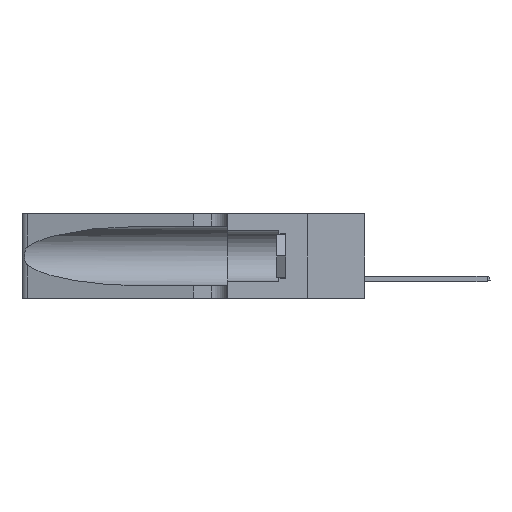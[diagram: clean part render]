
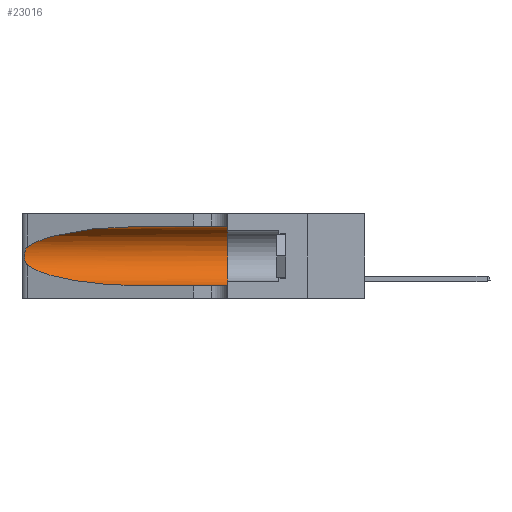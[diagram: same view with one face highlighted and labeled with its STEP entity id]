
A CAD part, left-side view. The second image highlights one B-rep face of the part: STEP entity #23016.
In plain terms, the highlighted cylindrical face has radius 3.308 mm (diameter 6.617 mm), a partial arc.
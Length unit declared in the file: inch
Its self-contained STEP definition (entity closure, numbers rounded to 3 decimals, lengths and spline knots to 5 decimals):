
#11 = EDGE_LOOP ( 'NONE', ( #14268, #11052, #5987, #9031, #28122, #39845 ) ) ;
#820 = CIRCLE ( 'NONE', #30884, 0.13025 ) ;
#2294 =( BOUNDED_CURVE ( )  B_SPLINE_CURVE ( 3, ( #7659, #23607, #17549, #39515 ),
 .UNSPECIFIED., .F., .F. ) 
 B_SPLINE_CURVE_WITH_KNOTS ( ( 4, 4 ),
 ( 1.5708, 2.84003 ),
 .UNSPECIFIED. ) 
 CURVE ( )  GEOMETRIC_REPRESENTATION_ITEM ( )  RATIONAL_B_SPLINE_CURVE ( ( 1., 0.87, 0.87, 1. ) ) 
 REPRESENTATION_ITEM ( '' )  );
#2702 = CARTESIAN_POINT ( 'NONE',  ( 0.25487, 1.22718, 0.14631 ) ) ;
#5159 = VERTEX_POINT ( 'NONE', #16169 ) ;
#5179 = CARTESIAN_POINT ( 'NONE',  ( 0.2373, 1.15595, 0.08982 ) ) ;
#5259 = CARTESIAN_POINT ( 'NONE',  ( 0.1305, 0.35, 0.185 ) ) ;
#5987 = ORIENTED_EDGE ( 'NONE', *, *, #15697, .T. ) ;
#7659 = CARTESIAN_POINT ( 'NONE',  ( 0.1305, 0.72297, 0.31525 ) ) ;
#9031 = ORIENTED_EDGE ( 'NONE', *, *, #18591, .T. ) ;
#10205 = CARTESIAN_POINT ( 'NONE',  ( 0.1305, 0.35, 0.31525 ) ) ;
#11052 = ORIENTED_EDGE ( 'NONE', *, *, #32203, .T. ) ;
#11164 = DIRECTION ( 'NONE',  ( 0., -1., 0. ) ) ;
#11564 = DIRECTION ( 'NONE',  ( 0., 0., 1. ) ) ;
#11741 = CARTESIAN_POINT ( 'NONE',  ( 0.25555, 1.22994, 0.2215 ) ) ;
#11879 = CARTESIAN_POINT ( 'NONE',  ( 0.25487, 1.22718, 0.22369 ) ) ;
#12000 = CARTESIAN_POINT ( 'NONE',  ( 0.26017, 1.23833, 0.17102 ) ) ;
#12102 = CARTESIAN_POINT ( 'NONE',  ( 0.1305, 1.61858, 0.31525 ) ) ;
#12310 = LINE ( 'NONE', #12102, #27990 ) ;
#13757 = CARTESIAN_POINT ( 'NONE',  ( 0.1305, 1.61858, 0.185 ) ) ;
#14212 = CARTESIAN_POINT ( 'NONE',  ( 0.25487, 1.22718, 0.14631 ) ) ;
#14268 = ORIENTED_EDGE ( 'NONE', *, *, #34778, .T. ) ;
#14655 = CARTESIAN_POINT ( 'NONE',  ( 0.25487, 1.22718, 0.22369 ) ) ;
#14999 = CARTESIAN_POINT ( 'NONE',  ( 0.25787, 1.23484, 0.2124 ) ) ;
#15697 = EDGE_CURVE ( 'NONE', #16358, #5159, #36166, .T. ) ;
#16169 = CARTESIAN_POINT ( 'NONE',  ( 0.1305, 0.72297, 0.05475 ) ) ;
#16358 = VERTEX_POINT ( 'NONE', #28517 ) ;
#17189 = VERTEX_POINT ( 'NONE', #31794 ) ;
#17332 = DIRECTION ( 'NONE',  ( 0., -1., 0. ) ) ;
#17549 = CARTESIAN_POINT ( 'NONE',  ( 0.2373, 1.15595, 0.28018 ) ) ;
#18153 = CARTESIAN_POINT ( 'NONE',  ( 0.26018, 1.23835, 0.19895 ) ) ;
#18591 = EDGE_CURVE ( 'NONE', #5159, #26201, #21809, .T. ) ;
#19627 = VERTEX_POINT ( 'NONE', #14655 ) ;
#20227 = DIRECTION ( 'NONE',  ( 0., 0., -1. ) ) ;
#21809 = LINE ( 'NONE', #29903, #26184 ) ;
#23016 = ADVANCED_FACE ( 'NONE', ( #27848 ), #32179, .F. ) ;
#23607 = CARTESIAN_POINT ( 'NONE',  ( 0.18966, 0.96281, 0.31525 ) ) ;
#24338 = CARTESIAN_POINT ( 'NONE',  ( 0.25639, 1.23184, 0.21858 ) ) ;
#24468 = CARTESIAN_POINT ( 'NONE',  ( 0.26075, 1.23896, 0.19203 ) ) ;
#24560 = AXIS2_PLACEMENT_3D ( 'NONE', #13757, #17332, #20227 ) ;
#24887 = VERTEX_POINT ( 'NONE', #10205 ) ;
#25396 = EDGE_CURVE ( 'NONE', #24887, #26201, #820, .T. ) ;
#25606 = CARTESIAN_POINT ( 'NONE',  ( 0.1305, 0.35, 0.05475 ) ) ;
#26184 = VECTOR ( 'NONE', #11164, 39.37008 ) ;
#26201 = VERTEX_POINT ( 'NONE', #25606 ) ;
#27079 = CARTESIAN_POINT ( 'NONE',  ( 0.1305, 0.72297, 0.05475 ) ) ;
#27152 = DIRECTION ( 'NONE',  ( 0., 1., 0. ) ) ;
#27599 = CARTESIAN_POINT ( 'NONE',  ( 0.26075, 1.23896, 0.178 ) ) ;
#27848 = FACE_OUTER_BOUND ( 'NONE', #11, .T. ) ;
#27990 = VECTOR ( 'NONE', #31357, 39.37008 ) ;
#28122 = ORIENTED_EDGE ( 'NONE', *, *, #25396, .F. ) ;
#28517 = CARTESIAN_POINT ( 'NONE',  ( 0.25487, 1.22718, 0.14631 ) ) ;
#28623 = EDGE_CURVE ( 'NONE', #17189, #24887, #12310, .T. ) ;
#28645 = CARTESIAN_POINT ( 'NONE',  ( 0.25789, 1.23486, 0.15765 ) ) ;
#29903 = CARTESIAN_POINT ( 'NONE',  ( 0.1305, 1.61858, 0.05475 ) ) ;
#30884 = AXIS2_PLACEMENT_3D ( 'NONE', #5259, #27152, #11564 ) ;
#31357 = DIRECTION ( 'NONE',  ( 0., -1., 0. ) ) ;
#31794 = CARTESIAN_POINT ( 'NONE',  ( 0.1305, 0.72297, 0.31525 ) ) ;
#32179 = CYLINDRICAL_SURFACE ( 'NONE', #24560, 0.13025 ) ;
#32203 = EDGE_CURVE ( 'NONE', #19627, #16358, #36932, .T. ) ;
#33867 = CARTESIAN_POINT ( 'NONE',  ( 0.25856, 1.23593, 0.16098 ) ) ;
#34778 = EDGE_CURVE ( 'NONE', #17189, #19627, #2294, .T. ) ;
#36166 =( BOUNDED_CURVE ( )  B_SPLINE_CURVE ( 3, ( #14212, #5179, #36213, #27079 ),
 .UNSPECIFIED., .F., .T. ) 
 B_SPLINE_CURVE_WITH_KNOTS ( ( 4, 4 ),
 ( 3.44316, 4.71239 ),
 .UNSPECIFIED. ) 
 CURVE ( )  GEOMETRIC_REPRESENTATION_ITEM ( )  RATIONAL_B_SPLINE_CURVE ( ( 1., 0.87, 0.87, 1. ) ) 
 REPRESENTATION_ITEM ( '' )  );
#36213 = CARTESIAN_POINT ( 'NONE',  ( 0.18966, 0.96281, 0.05475 ) ) ;
#36896 = CARTESIAN_POINT ( 'NONE',  ( 0.25854, 1.2359, 0.20912 ) ) ;
#36932 = B_SPLINE_CURVE_WITH_KNOTS ( 'NONE', 3,
 ( #11879, #11741, #24338, #14999, #36896, #18153, #24468, #27599, #12000, #33867, #28645, #38924, #37489, #2702 ),
 .UNSPECIFIED., .F., .F.,
 ( 4, 2, 2, 2, 2, 2, 4 ),
 ( 0., 0.00027, 0.00053, 0.00107, 0.0016, 0.00187, 0.00214 ),
 .UNSPECIFIED. ) ;
#37489 = CARTESIAN_POINT ( 'NONE',  ( 0.25555, 1.22993, 0.14849 ) ) ;
#38924 = CARTESIAN_POINT ( 'NONE',  ( 0.25639, 1.23186, 0.15144 ) ) ;
#39515 = CARTESIAN_POINT ( 'NONE',  ( 0.25487, 1.22718, 0.22369 ) ) ;
#39845 = ORIENTED_EDGE ( 'NONE', *, *, #28623, .F. ) ;
